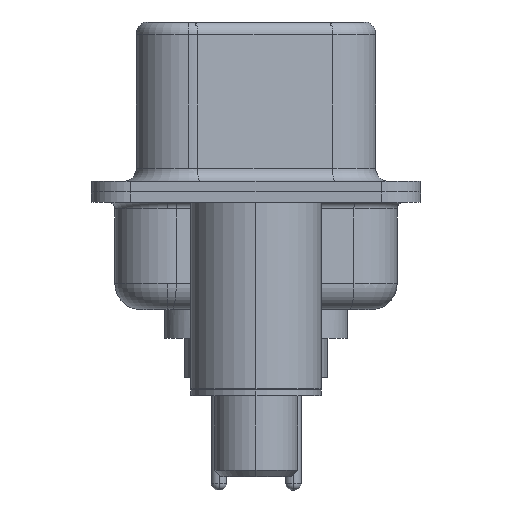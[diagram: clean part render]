
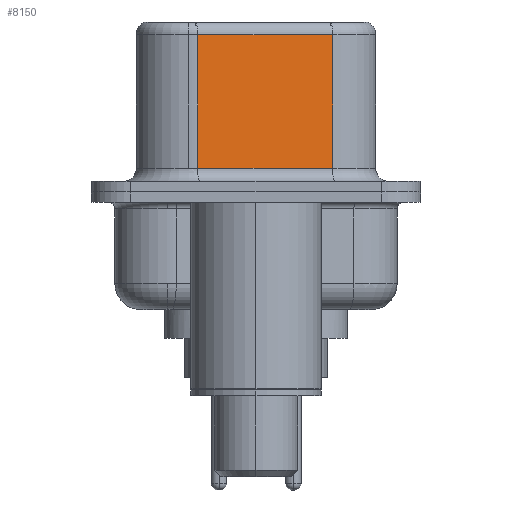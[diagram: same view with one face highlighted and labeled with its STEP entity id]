
A CAD part, left-side view. The second image highlights one B-rep face of the part: STEP entity #8150.
In plain terms, the highlighted planar face has unit normal (-0.985, -0.174, 0).
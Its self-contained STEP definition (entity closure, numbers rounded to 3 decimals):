
#96 = CARTESIAN_POINT ( 'NONE',  ( 4.58, -2.927, 0.9 ) ) ;
#225 = VERTEX_POINT ( 'NONE', #20353 ) ;
#758 = CARTESIAN_POINT ( 'NONE',  ( 4.58, -2.927, 6.52 ) ) ;
#2272 = LINE ( 'NONE', #23447, #22762 ) ;
#2711 = EDGE_LOOP ( 'NONE', ( #6473, #11853, #10607, #4102 ) ) ;
#3686 = EDGE_CURVE ( 'NONE', #225, #15065, #6892, .T. ) ;
#3694 = DIRECTION ( 'NONE',  ( 0., 0., -1. ) ) ;
#4036 = DIRECTION ( 'NONE',  ( -0.174, 0.985, 0. ) ) ;
#4102 = ORIENTED_EDGE ( 'NONE', *, *, #3686, .T. ) ;
#6264 = VECTOR ( 'NONE', #16634, 1000. ) ;
#6473 = ORIENTED_EDGE ( 'NONE', *, *, #15626, .F. ) ;
#6538 = AXIS2_PLACEMENT_3D ( 'NONE', #758, #10683, #24584 ) ;
#6892 = LINE ( 'NONE', #96, #6264 ) ;
#7108 = CARTESIAN_POINT ( 'NONE',  ( 3.67, 2.233, 6.02 ) ) ;
#7887 = EDGE_CURVE ( 'NONE', #18695, #9216, #20817, .T. ) ;
#7918 = CARTESIAN_POINT ( 'NONE',  ( 4.58, -2.927, 6.02 ) ) ;
#8150 = ADVANCED_FACE ( 'NONE', ( #11176 ), #18558, .F. ) ;
#8702 = CARTESIAN_POINT ( 'NONE',  ( 4.58, -2.927, 0.9 ) ) ;
#9216 = VERTEX_POINT ( 'NONE', #7108 ) ;
#10607 = ORIENTED_EDGE ( 'NONE', *, *, #14723, .T. ) ;
#10683 = DIRECTION ( 'NONE',  ( 0.985, 0.174, 0. ) ) ;
#11176 = FACE_OUTER_BOUND ( 'NONE', #2711, .T. ) ;
#11212 = VECTOR ( 'NONE', #18441, 1000. ) ;
#11853 = ORIENTED_EDGE ( 'NONE', *, *, #7887, .T. ) ;
#14143 = CARTESIAN_POINT ( 'NONE',  ( 4.58, -2.927, 6.02 ) ) ;
#14723 = EDGE_CURVE ( 'NONE', #9216, #225, #2272, .T. ) ;
#15065 = VERTEX_POINT ( 'NONE', #8702 ) ;
#15529 = VECTOR ( 'NONE', #4036, 1000. ) ;
#15626 = EDGE_CURVE ( 'NONE', #18695, #15065, #22410, .T. ) ;
#16634 = DIRECTION ( 'NONE',  ( 0.174, -0.985, 0. ) ) ;
#18441 = DIRECTION ( 'NONE',  ( 0., 0., -1. ) ) ;
#18558 = PLANE ( 'NONE',  #6538 ) ;
#18695 = VERTEX_POINT ( 'NONE', #14143 ) ;
#20353 = CARTESIAN_POINT ( 'NONE',  ( 3.67, 2.233, 0.9 ) ) ;
#20817 = LINE ( 'NONE', #7918, #15529 ) ;
#22410 = LINE ( 'NONE', #22477, #11212 ) ;
#22477 = CARTESIAN_POINT ( 'NONE',  ( 4.58, -2.927, 6.52 ) ) ;
#22762 = VECTOR ( 'NONE', #3694, 1000. ) ;
#23447 = CARTESIAN_POINT ( 'NONE',  ( 3.67, 2.233, 6.52 ) ) ;
#24584 = DIRECTION ( 'NONE',  ( -0.174, 0.985, 0. ) ) ;
